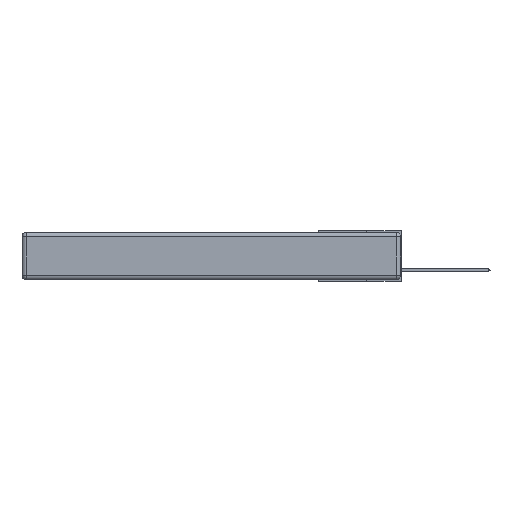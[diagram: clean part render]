
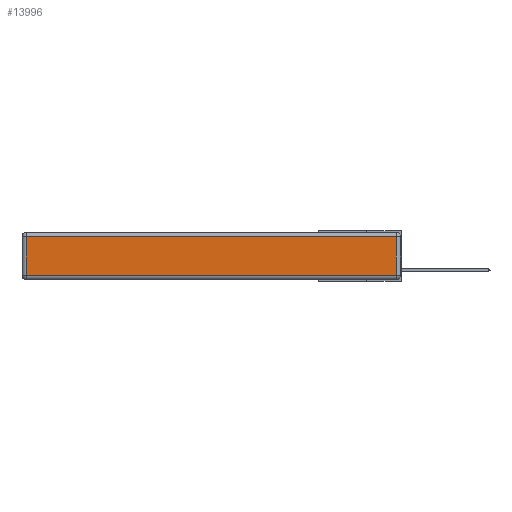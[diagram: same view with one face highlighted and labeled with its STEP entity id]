
A CAD part, left-side view. The second image highlights one B-rep face of the part: STEP entity #13996.
In plain terms, the highlighted planar face has unit normal (-1, 0, 0).
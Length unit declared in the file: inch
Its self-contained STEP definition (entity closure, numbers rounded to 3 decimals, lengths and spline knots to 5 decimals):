
#36 = CARTESIAN_POINT ( 'NONE',  ( 0., 0.03, -0.313 ) ) ;
#178 = ORIENTED_EDGE ( 'NONE', *, *, #7706, .T. ) ;
#812 = VERTEX_POINT ( 'NONE', #36 ) ;
#898 = VECTOR ( 'NONE', #9693, 39.37008 ) ;
#2055 = PLANE ( 'NONE',  #2673 ) ;
#2123 = VERTEX_POINT ( 'NONE', #2376 ) ;
#2376 = CARTESIAN_POINT ( 'NONE',  ( 0., 0.03, -0.03 ) ) ;
#2611 = CARTESIAN_POINT ( 'NONE',  ( 0., 2.72, -0.343 ) ) ;
#2673 = AXIS2_PLACEMENT_3D ( 'NONE', #12501, #7843, #7251 ) ;
#2732 = LINE ( 'NONE', #2885, #14140 ) ;
#2885 = CARTESIAN_POINT ( 'NONE',  ( 0., 0.03, -0.343 ) ) ;
#2955 = ORIENTED_EDGE ( 'NONE', *, *, #12919, .T. ) ;
#3129 = EDGE_CURVE ( 'NONE', #812, #2123, #2732, .T. ) ;
#4020 = DIRECTION ( 'NONE',  ( 0., 0., 1. ) ) ;
#5233 = LINE ( 'NONE', #11694, #11979 ) ;
#6070 = LINE ( 'NONE', #2611, #898 ) ;
#6290 = DIRECTION ( 'NONE',  ( 0., 1., 0. ) ) ;
#6894 = EDGE_CURVE ( 'NONE', #2123, #8160, #14263, .T. ) ;
#7251 = DIRECTION ( 'NONE',  ( 0., 0., 1. ) ) ;
#7390 = CARTESIAN_POINT ( 'NONE',  ( 0., 2.72, -0.313 ) ) ;
#7689 = EDGE_LOOP ( 'NONE', ( #2955, #14240, #12194, #178 ) ) ;
#7706 = EDGE_CURVE ( 'NONE', #8160, #8007, #6070, .T. ) ;
#7843 = DIRECTION ( 'NONE',  ( -1., 0., 0. ) ) ;
#8007 = VERTEX_POINT ( 'NONE', #7390 ) ;
#8160 = VERTEX_POINT ( 'NONE', #9834 ) ;
#9434 = FACE_OUTER_BOUND ( 'NONE', #7689, .T. ) ;
#9441 = DIRECTION ( 'NONE',  ( 0., -1., 0. ) ) ;
#9693 = DIRECTION ( 'NONE',  ( 0., 0., -1. ) ) ;
#9834 = CARTESIAN_POINT ( 'NONE',  ( 0., 2.72, -0.03 ) ) ;
#11694 = CARTESIAN_POINT ( 'NONE',  ( 0., 0., -0.313 ) ) ;
#11979 = VECTOR ( 'NONE', #9441, 39.37008 ) ;
#12194 = ORIENTED_EDGE ( 'NONE', *, *, #6894, .T. ) ;
#12501 = CARTESIAN_POINT ( 'NONE',  ( 0., 0., -0.343 ) ) ;
#12519 = VECTOR ( 'NONE', #6290, 39.37008 ) ;
#12919 = EDGE_CURVE ( 'NONE', #8007, #812, #5233, .T. ) ;
#13265 = CARTESIAN_POINT ( 'NONE',  ( 0., 2.75, -0.03 ) ) ;
#13996 = ADVANCED_FACE ( 'NONE', ( #9434 ), #2055, .T. ) ;
#14140 = VECTOR ( 'NONE', #4020, 39.37008 ) ;
#14240 = ORIENTED_EDGE ( 'NONE', *, *, #3129, .T. ) ;
#14263 = LINE ( 'NONE', #13265, #12519 ) ;
